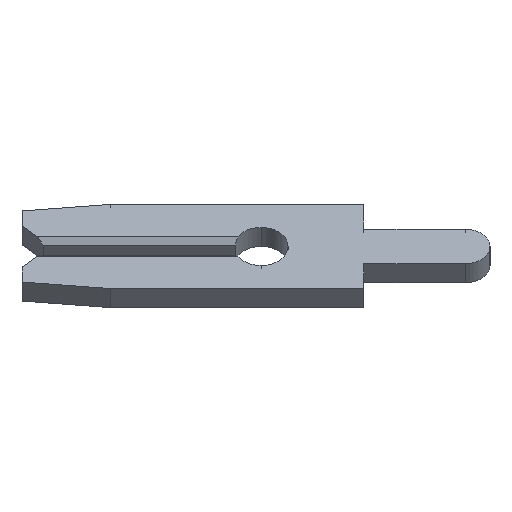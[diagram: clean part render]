
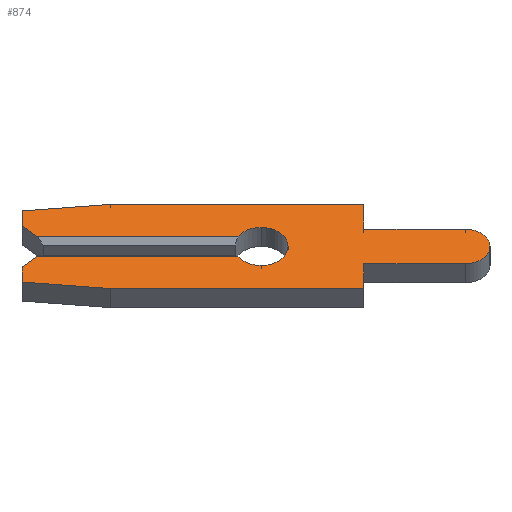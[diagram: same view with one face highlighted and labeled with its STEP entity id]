
A CAD part, left-side view. The second image highlights one B-rep face of the part: STEP entity #874.
In plain terms, the highlighted face is planar.
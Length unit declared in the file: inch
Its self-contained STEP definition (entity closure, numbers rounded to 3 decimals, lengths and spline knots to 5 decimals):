
#10 = ORIENTED_EDGE ( 'NONE', *, *, #304, .F. ) ;
#12 = ORIENTED_EDGE ( 'NONE', *, *, #412, .F. ) ;
#20 = CARTESIAN_POINT ( 'NONE',  ( -0.013, -0.099, -0.0235 ) ) ;
#24 = VERTEX_POINT ( 'NONE', #710 ) ;
#52 = DIRECTION ( 'NONE',  ( 0., 1., 0. ) ) ;
#61 = ORIENTED_EDGE ( 'NONE', *, *, #500, .F. ) ;
#72 = CARTESIAN_POINT ( 'NONE',  ( -0.013, 0.231, 0.013 ) ) ;
#89 = ORIENTED_EDGE ( 'NONE', *, *, #310, .F. ) ;
#112 = CARTESIAN_POINT ( 'NONE',  ( -0.013, -0.099, 0.0575 ) ) ;
#116 = DIRECTION ( 'NONE',  ( 0., 0., -1. ) ) ;
#128 = DIRECTION ( 'NONE',  ( -1., 0., 0. ) ) ;
#131 = EDGE_CURVE ( 'NONE', #24, #1066, #1062, .T. ) ;
#146 = ORIENTED_EDGE ( 'NONE', *, *, #399, .F. ) ;
#162 = VECTOR ( 'NONE', #954, 39.37008 ) ;
#164 = CARTESIAN_POINT ( 'NONE',  ( -0.013, 0., 0. ) ) ;
#166 = VERTEX_POINT ( 'NONE', #933 ) ;
#178 = LINE ( 'NONE', #750, #790 ) ;
#192 = VECTOR ( 'NONE', #213, 39.37008 ) ;
#210 = EDGE_LOOP ( 'NONE', ( #437, #12, #785, #875, #526, #61, #89, #625, #10, #726, #146, #1156, #865, #547, #960, #1251, #1224, #375 ) ) ;
#213 = DIRECTION ( 'NONE',  ( 0., 0.995, 0.105 ) ) ;
#214 = VECTOR ( 'NONE', #523, 39.37008 ) ;
#232 = VERTEX_POINT ( 'NONE', #1028 ) ;
#250 = LINE ( 'NONE', #900, #192 ) ;
#261 = CARTESIAN_POINT ( 'NONE',  ( -0.013, -0.099, 0.0575 ) ) ;
#265 = VERTEX_POINT ( 'NONE', #1140 ) ;
#269 = EDGE_CURVE ( 'NONE', #297, #1024, #512, .T. ) ;
#273 = CARTESIAN_POINT ( 'NONE',  ( -0.013, 0.231, -0.028 ) ) ;
#276 = VERTEX_POINT ( 'NONE', #740 ) ;
#282 = EDGE_CURVE ( 'NONE', #1024, #24, #1149, .T. ) ;
#284 = DIRECTION ( 'NONE',  ( 0., 0., 1. ) ) ;
#290 = DIRECTION ( 'NONE',  ( 0., 0.707, 0.707 ) ) ;
#297 = VERTEX_POINT ( 'NONE', #623 ) ;
#298 = CARTESIAN_POINT ( 'NONE',  ( -0.013, -0.099, -0.0575 ) ) ;
#299 = LINE ( 'NONE', #112, #422 ) ;
#304 = EDGE_CURVE ( 'NONE', #752, #861, #958, .T. ) ;
#310 = EDGE_CURVE ( 'NONE', #704, #647, #585, .T. ) ;
#315 = CARTESIAN_POINT ( 'NONE',  ( -0.013, 0., 0. ) ) ;
#322 = DIRECTION ( 'NONE',  ( 0., -1., 0. ) ) ;
#324 = EDGE_CURVE ( 'NONE', #265, #276, #178, .T. ) ;
#334 = CARTESIAN_POINT ( 'NONE',  ( -0.013, -0.099, 0.0235 ) ) ;
#354 = DIRECTION ( 'NONE',  ( 0., 1., 0. ) ) ;
#368 = CARTESIAN_POINT ( 'NONE',  ( -0.013, 0., 0. ) ) ;
#372 = DIRECTION ( 'NONE',  ( -1., 0., 0. ) ) ;
#375 = ORIENTED_EDGE ( 'NONE', *, *, #657, .F. ) ;
#384 = CARTESIAN_POINT ( 'NONE',  ( -0.013, -0.1975, 0. ) ) ;
#394 = VERTEX_POINT ( 'NONE', #858 ) ;
#397 = CARTESIAN_POINT ( 'NONE',  ( -0.013, 0.2105, 0.0075 ) ) ;
#399 = EDGE_CURVE ( 'NONE', #394, #961, #1058, .T. ) ;
#408 = LINE ( 'NONE', #397, #471 ) ;
#412 = EDGE_CURVE ( 'NONE', #1131, #166, #493, .T. ) ;
#422 = VECTOR ( 'NONE', #591, 39.37008 ) ;
#424 = AXIS2_PLACEMENT_3D ( 'NONE', #384, #672, #284 ) ;
#427 = PLANE ( 'NONE',  #926 ) ;
#437 = ORIENTED_EDGE ( 'NONE', *, *, #639, .T. ) ;
#441 = CARTESIAN_POINT ( 'NONE',  ( -0.013, 0.231, 0.028 ) ) ;
#456 = CARTESIAN_POINT ( 'NONE',  ( -0.013, 0., 0.026 ) ) ;
#458 = CARTESIAN_POINT ( 'NONE',  ( -0.013, 0.2105, -0.0075 ) ) ;
#462 = DIRECTION ( 'NONE',  ( 0., 0., -1. ) ) ;
#471 = VECTOR ( 'NONE', #290, 39.37008 ) ;
#477 = EDGE_CURVE ( 'NONE', #629, #1131, #528, .T. ) ;
#479 = LINE ( 'NONE', #495, #1023 ) ;
#493 = CIRCLE ( 'NONE', #711, 0.026 ) ;
#495 = CARTESIAN_POINT ( 'NONE',  ( -0.013, -0.099, -0.0575 ) ) ;
#500 = EDGE_CURVE ( 'NONE', #647, #265, #1225, .T. ) ;
#512 = LINE ( 'NONE', #441, #214 ) ;
#523 = DIRECTION ( 'NONE',  ( 0., 0., 1. ) ) ;
#525 = LINE ( 'NONE', #334, #993 ) ;
#526 = ORIENTED_EDGE ( 'NONE', *, *, #324, .F. ) ;
#528 = CIRCLE ( 'NONE', #652, 0.026 ) ;
#547 = ORIENTED_EDGE ( 'NONE', *, *, #702, .F. ) ;
#585 = LINE ( 'NONE', #1126, #667 ) ;
#591 = DIRECTION ( 'NONE',  ( 0., 0., -1. ) ) ;
#610 = VERTEX_POINT ( 'NONE', #763 ) ;
#620 = EDGE_CURVE ( 'NONE', #661, #394, #758, .T. ) ;
#623 = CARTESIAN_POINT ( 'NONE',  ( -0.013, 0.231, 0.028 ) ) ;
#625 = ORIENTED_EDGE ( 'NONE', *, *, #764, .F. ) ;
#629 = VERTEX_POINT ( 'NONE', #878 ) ;
#632 = DIRECTION ( 'NONE',  ( 0., -0.995, 0.105 ) ) ;
#634 = VECTOR ( 'NONE', #354, 39.37008 ) ;
#639 = EDGE_CURVE ( 'NONE', #232, #166, #950, .T. ) ;
#640 = DIRECTION ( 'NONE',  ( 0., -1., 0. ) ) ;
#647 = VERTEX_POINT ( 'NONE', #273 ) ;
#652 = AXIS2_PLACEMENT_3D ( 'NONE', #368, #1055, #462 ) ;
#657 = EDGE_CURVE ( 'NONE', #232, #297, #408, .T. ) ;
#661 = VERTEX_POINT ( 'NONE', #690 ) ;
#665 = DIRECTION ( 'NONE',  ( 0., -1., 0. ) ) ;
#667 = VECTOR ( 'NONE', #957, 39.37008 ) ;
#672 = DIRECTION ( 'NONE',  ( 1., 0., 0. ) ) ;
#690 = CARTESIAN_POINT ( 'NONE',  ( -0.013, -0.1975, 0.0235 ) ) ;
#702 = EDGE_CURVE ( 'NONE', #1066, #610, #299, .T. ) ;
#704 = VERTEX_POINT ( 'NONE', #804 ) ;
#710 = CARTESIAN_POINT ( 'NONE',  ( -0.013, 0.146, 0.0575 ) ) ;
#711 = AXIS2_PLACEMENT_3D ( 'NONE', #164, #372, #1061 ) ;
#717 = CARTESIAN_POINT ( 'NONE',  ( -0.013, 0., 0. ) ) ;
#726 = ORIENTED_EDGE ( 'NONE', *, *, #797, .F. ) ;
#740 = CARTESIAN_POINT ( 'NONE',  ( -0.013, 0.02252, -0.013 ) ) ;
#750 = CARTESIAN_POINT ( 'NONE',  ( -0.013, 0., -0.013 ) ) ;
#752 = VERTEX_POINT ( 'NONE', #298 ) ;
#758 = CIRCLE ( 'NONE', #424, 0.0235 ) ;
#763 = CARTESIAN_POINT ( 'NONE',  ( -0.013, -0.099, 0.0235 ) ) ;
#764 = EDGE_CURVE ( 'NONE', #861, #704, #250, .T. ) ;
#785 = ORIENTED_EDGE ( 'NONE', *, *, #477, .F. ) ;
#790 = VECTOR ( 'NONE', #640, 39.37008 ) ;
#797 = EDGE_CURVE ( 'NONE', #961, #752, #479, .T. ) ;
#801 = DIRECTION ( 'NONE',  ( 0., -1., 0. ) ) ;
#804 = CARTESIAN_POINT ( 'NONE',  ( -0.013, 0.231, -0.04857 ) ) ;
#810 = CARTESIAN_POINT ( 'NONE',  ( -0.013, 0.231, 0.04857 ) ) ;
#821 = DIRECTION ( 'NONE',  ( 0., 0., -1. ) ) ;
#834 = VECTOR ( 'NONE', #801, 39.37008 ) ;
#854 = FACE_OUTER_BOUND ( 'NONE', #210, .T. ) ;
#858 = CARTESIAN_POINT ( 'NONE',  ( -0.013, -0.1975, -0.0235 ) ) ;
#861 = VERTEX_POINT ( 'NONE', #884 ) ;
#864 = EDGE_CURVE ( 'NONE', #610, #661, #525, .T. ) ;
#865 = ORIENTED_EDGE ( 'NONE', *, *, #864, .F. ) ;
#874 = ADVANCED_FACE ( 'NONE', ( #854 ), #427, .F. ) ;
#875 = ORIENTED_EDGE ( 'NONE', *, *, #1022, .F. ) ;
#878 = CARTESIAN_POINT ( 'NONE',  ( -0.013, 0., -0.026 ) ) ;
#884 = CARTESIAN_POINT ( 'NONE',  ( -0.013, 0.146, -0.0575 ) ) ;
#900 = CARTESIAN_POINT ( 'NONE',  ( -0.013, 0.231, -0.04857 ) ) ;
#926 = AXIS2_PLACEMENT_3D ( 'NONE', #315, #1021, #821 ) ;
#930 = CARTESIAN_POINT ( 'NONE',  ( -0.013, 0.146, -0.0575 ) ) ;
#933 = CARTESIAN_POINT ( 'NONE',  ( -0.013, 0.02252, 0.013 ) ) ;
#950 = LINE ( 'NONE', #72, #1179 ) ;
#954 = DIRECTION ( 'NONE',  ( 0., -0.707, 0.707 ) ) ;
#957 = DIRECTION ( 'NONE',  ( 0., 0., 1. ) ) ;
#958 = LINE ( 'NONE', #930, #1081 ) ;
#960 = ORIENTED_EDGE ( 'NONE', *, *, #131, .F. ) ;
#961 = VERTEX_POINT ( 'NONE', #20 ) ;
#993 = VECTOR ( 'NONE', #322, 39.37008 ) ;
#997 = DIRECTION ( 'NONE',  ( 0., 0., -1. ) ) ;
#1021 = DIRECTION ( 'NONE',  ( 1., 0., 0. ) ) ;
#1022 = EDGE_CURVE ( 'NONE', #276, #629, #1208, .T. ) ;
#1023 = VECTOR ( 'NONE', #997, 39.37008 ) ;
#1024 = VERTEX_POINT ( 'NONE', #810 ) ;
#1028 = CARTESIAN_POINT ( 'NONE',  ( -0.013, 0.216, 0.013 ) ) ;
#1055 = DIRECTION ( 'NONE',  ( -1., 0., 0. ) ) ;
#1057 = AXIS2_PLACEMENT_3D ( 'NONE', #717, #128, #116 ) ;
#1058 = LINE ( 'NONE', #1157, #634 ) ;
#1061 = DIRECTION ( 'NONE',  ( 0., 0., -1. ) ) ;
#1062 = LINE ( 'NONE', #1214, #834 ) ;
#1066 = VERTEX_POINT ( 'NONE', #261 ) ;
#1081 = VECTOR ( 'NONE', #52, 39.37008 ) ;
#1085 = VECTOR ( 'NONE', #632, 39.37008 ) ;
#1126 = CARTESIAN_POINT ( 'NONE',  ( -0.013, 0.231, -0.028 ) ) ;
#1129 = CARTESIAN_POINT ( 'NONE',  ( -0.013, 0.231, 0.04857 ) ) ;
#1131 = VERTEX_POINT ( 'NONE', #456 ) ;
#1140 = CARTESIAN_POINT ( 'NONE',  ( -0.013, 0.216, -0.013 ) ) ;
#1149 = LINE ( 'NONE', #1129, #1085 ) ;
#1156 = ORIENTED_EDGE ( 'NONE', *, *, #620, .F. ) ;
#1157 = CARTESIAN_POINT ( 'NONE',  ( -0.013, -0.099, -0.0235 ) ) ;
#1179 = VECTOR ( 'NONE', #665, 39.37008 ) ;
#1208 = CIRCLE ( 'NONE', #1057, 0.026 ) ;
#1214 = CARTESIAN_POINT ( 'NONE',  ( -0.013, 0.146, 0.0575 ) ) ;
#1224 = ORIENTED_EDGE ( 'NONE', *, *, #269, .F. ) ;
#1225 = LINE ( 'NONE', #458, #162 ) ;
#1251 = ORIENTED_EDGE ( 'NONE', *, *, #282, .F. ) ;
